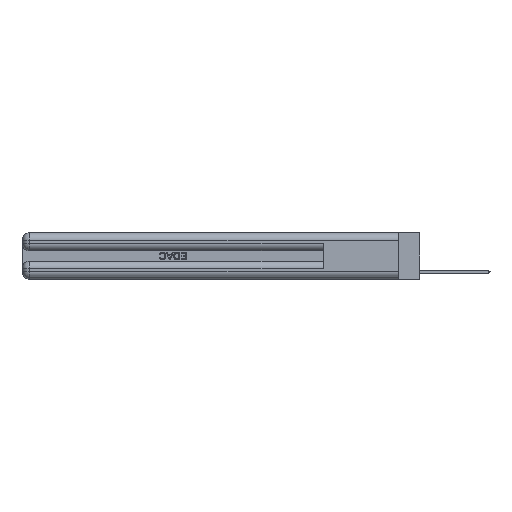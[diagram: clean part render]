
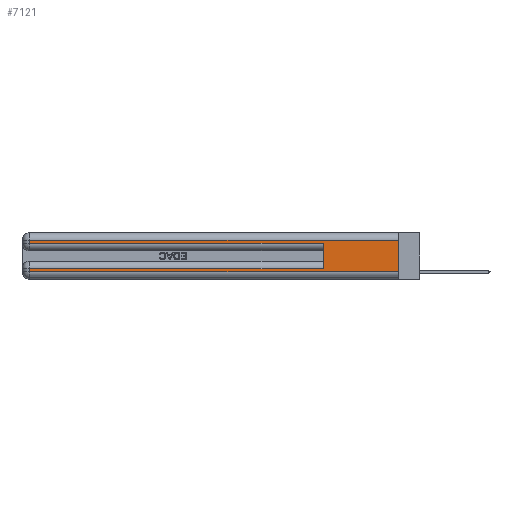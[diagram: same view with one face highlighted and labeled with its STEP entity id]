
A CAD part, left-side view. The second image highlights one B-rep face of the part: STEP entity #7121.
In plain terms, the highlighted planar face has unit normal (-1, 0, 0).
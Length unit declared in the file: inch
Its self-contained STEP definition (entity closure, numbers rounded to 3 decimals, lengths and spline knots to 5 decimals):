
#192 = EDGE_CURVE ( 'NONE', #31841, #25442, #28333, .T. ) ;
#536 = EDGE_LOOP ( 'NONE', ( #731, #6446, #725, #29490, #27565, #7237, #13843, #13928 ) ) ;
#556 = VECTOR ( 'NONE', #26611, 39.37008 ) ;
#725 = ORIENTED_EDGE ( 'NONE', *, *, #22285, .T. ) ;
#731 = ORIENTED_EDGE ( 'NONE', *, *, #3138, .F. ) ;
#1010 = AXIS2_PLACEMENT_3D ( 'NONE', #15517, #10452, #25166 ) ;
#1601 = VECTOR ( 'NONE', #15908, 39.37008 ) ;
#2103 = CARTESIAN_POINT ( 'NONE',  ( 0., 2.94, 0.06 ) ) ;
#2466 = VERTEX_POINT ( 'NONE', #22493 ) ;
#3138 = EDGE_CURVE ( 'NONE', #2466, #25442, #23926, .T. ) ;
#3516 = CARTESIAN_POINT ( 'NONE',  ( 0., 0., 0.285 ) ) ;
#3666 = DIRECTION ( 'NONE',  ( 0., 1., 0. ) ) ;
#3672 = CARTESIAN_POINT ( 'NONE',  ( 0., 0., 0.37 ) ) ;
#3775 = CARTESIAN_POINT ( 'NONE',  ( 0., 2.94, 0.285 ) ) ;
#4290 = CARTESIAN_POINT ( 'NONE',  ( 0., 2.94, 0.085 ) ) ;
#5193 = VECTOR ( 'NONE', #28525, 39.37008 ) ;
#5256 = VECTOR ( 'NONE', #24145, 39.37008 ) ;
#5884 = FACE_OUTER_BOUND ( 'NONE', #536, .T. ) ;
#5945 = CARTESIAN_POINT ( 'NONE',  ( 0., 0., 0.06 ) ) ;
#6446 = ORIENTED_EDGE ( 'NONE', *, *, #25045, .T. ) ;
#7121 = ADVANCED_FACE ( 'NONE', ( #5884 ), #20234, .F. ) ;
#7237 = ORIENTED_EDGE ( 'NONE', *, *, #17059, .T. ) ;
#8948 = CARTESIAN_POINT ( 'NONE',  ( 0., 2.94, 0.37 ) ) ;
#9438 = VECTOR ( 'NONE', #29541, 39.37008 ) ;
#10452 = DIRECTION ( 'NONE',  ( 1., 0., 0. ) ) ;
#11238 = VERTEX_POINT ( 'NONE', #3775 ) ;
#11863 = CARTESIAN_POINT ( 'NONE',  ( 0., 0.6, 0.285 ) ) ;
#13753 = VECTOR ( 'NONE', #3666, 39.37008 ) ;
#13843 = ORIENTED_EDGE ( 'NONE', *, *, #22239, .T. ) ;
#13928 = ORIENTED_EDGE ( 'NONE', *, *, #192, .T. ) ;
#14178 = LINE ( 'NONE', #16615, #5256 ) ;
#15517 = CARTESIAN_POINT ( 'NONE',  ( 0., 0., 0.37 ) ) ;
#15908 = DIRECTION ( 'NONE',  ( 0., -1., 0. ) ) ;
#16123 = LINE ( 'NONE', #29852, #9438 ) ;
#16287 = LINE ( 'NONE', #8948, #556 ) ;
#16615 = CARTESIAN_POINT ( 'NONE',  ( 0., 2.94, 0.37 ) ) ;
#17059 = EDGE_CURVE ( 'NONE', #24585, #18830, #31459, .T. ) ;
#18830 = VERTEX_POINT ( 'NONE', #4290 ) ;
#19633 = CARTESIAN_POINT ( 'NONE',  ( 0., 0.6, 0.085 ) ) ;
#20234 = PLANE ( 'NONE',  #1010 ) ;
#21148 = LINE ( 'NONE', #3516, #5193 ) ;
#22239 = EDGE_CURVE ( 'NONE', #18830, #31841, #16287, .T. ) ;
#22285 = EDGE_CURVE ( 'NONE', #27666, #11238, #14178, .T. ) ;
#22329 = EDGE_CURVE ( 'NONE', #24585, #29532, #16123, .T. ) ;
#22493 = CARTESIAN_POINT ( 'NONE',  ( 0., 0., 0.31 ) ) ;
#22528 = VECTOR ( 'NONE', #23068, 39.37008 ) ;
#22795 = EDGE_CURVE ( 'NONE', #11238, #29532, #21148, .T. ) ;
#23068 = DIRECTION ( 'NONE',  ( 0., 1., 0. ) ) ;
#23232 = LINE ( 'NONE', #23386, #22528 ) ;
#23350 = CARTESIAN_POINT ( 'NONE',  ( 0., 0., 0.06 ) ) ;
#23386 = CARTESIAN_POINT ( 'NONE',  ( 0., 0., 0.31 ) ) ;
#23589 = CARTESIAN_POINT ( 'NONE',  ( 0., 0., 0.085 ) ) ;
#23926 = LINE ( 'NONE', #3672, #24363 ) ;
#24145 = DIRECTION ( 'NONE',  ( 0., 0., -1. ) ) ;
#24363 = VECTOR ( 'NONE', #31134, 39.37008 ) ;
#24585 = VERTEX_POINT ( 'NONE', #19633 ) ;
#25045 = EDGE_CURVE ( 'NONE', #2466, #27666, #23232, .T. ) ;
#25067 = CARTESIAN_POINT ( 'NONE',  ( 0., 2.94, 0.31 ) ) ;
#25166 = DIRECTION ( 'NONE',  ( 0., 0., -1. ) ) ;
#25442 = VERTEX_POINT ( 'NONE', #23350 ) ;
#26611 = DIRECTION ( 'NONE',  ( 0., 0., -1. ) ) ;
#27565 = ORIENTED_EDGE ( 'NONE', *, *, #22329, .F. ) ;
#27666 = VERTEX_POINT ( 'NONE', #25067 ) ;
#28333 = LINE ( 'NONE', #5945, #1601 ) ;
#28525 = DIRECTION ( 'NONE',  ( 0., -1., 0. ) ) ;
#29490 = ORIENTED_EDGE ( 'NONE', *, *, #22795, .T. ) ;
#29532 = VERTEX_POINT ( 'NONE', #11863 ) ;
#29541 = DIRECTION ( 'NONE',  ( 0., 0., 1. ) ) ;
#29852 = CARTESIAN_POINT ( 'NONE',  ( 0., 0.6, 0.145 ) ) ;
#31134 = DIRECTION ( 'NONE',  ( 0., 0., -1. ) ) ;
#31459 = LINE ( 'NONE', #23589, #13753 ) ;
#31841 = VERTEX_POINT ( 'NONE', #2103 ) ;
